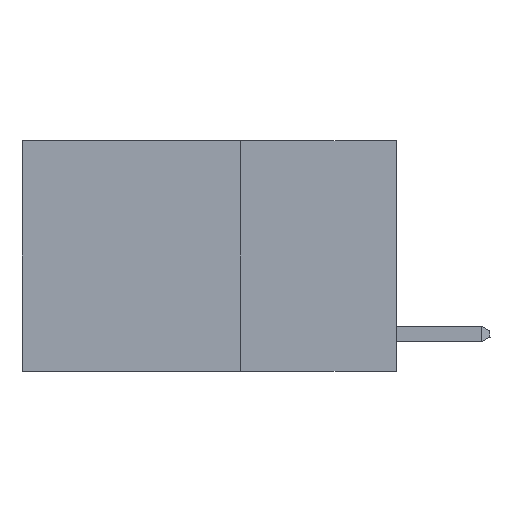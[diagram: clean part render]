
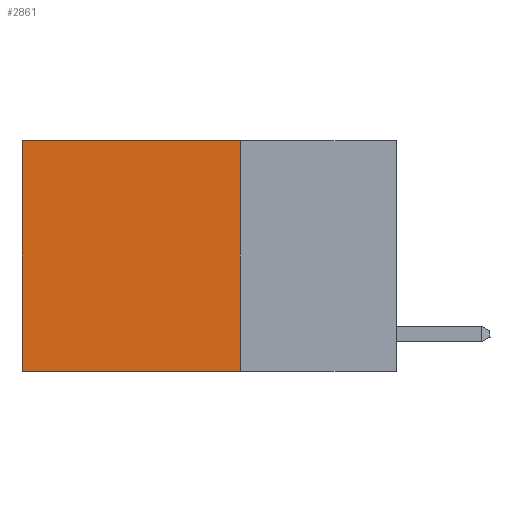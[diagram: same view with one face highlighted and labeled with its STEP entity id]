
A CAD part, left-side view. The second image highlights one B-rep face of the part: STEP entity #2861.
In plain terms, the highlighted planar face has unit normal (-1, 0, 0).
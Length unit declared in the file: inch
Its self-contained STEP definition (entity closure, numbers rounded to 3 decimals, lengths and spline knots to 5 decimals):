
#125 = VERTEX_POINT ( 'NONE', #4732 ) ;
#134 = LINE ( 'NONE', #2473, #5470 ) ;
#230 = ORIENTED_EDGE ( 'NONE', *, *, #5368, .F. ) ;
#691 = VERTEX_POINT ( 'NONE', #4814 ) ;
#1223 = LINE ( 'NONE', #2887, #5284 ) ;
#1435 = CARTESIAN_POINT ( 'NONE',  ( 0.2625, 0.25, -0.37 ) ) ;
#1844 = VERTEX_POINT ( 'NONE', #8013 ) ;
#2473 = CARTESIAN_POINT ( 'NONE',  ( 0.2625, 0.25, 0. ) ) ;
#2756 = LINE ( 'NONE', #1435, #7058 ) ;
#2855 = EDGE_CURVE ( 'NONE', #1844, #125, #134, .T. ) ;
#2861 = ADVANCED_FACE ( 'NONE', ( #9368 ), #5526, .F. ) ;
#2887 = CARTESIAN_POINT ( 'NONE',  ( 0.2625, 0.25, 0. ) ) ;
#3070 = DIRECTION ( 'NONE',  ( 0., 0., -1. ) ) ;
#3236 = CARTESIAN_POINT ( 'NONE',  ( 0.2625, 0.25, 0. ) ) ;
#3537 = EDGE_CURVE ( 'NONE', #691, #5918, #2756, .T. ) ;
#3665 = DIRECTION ( 'NONE',  ( 0., 1., 0. ) ) ;
#3879 = CARTESIAN_POINT ( 'NONE',  ( 0.2625, 0.6, 0. ) ) ;
#3887 = AXIS2_PLACEMENT_3D ( 'NONE', #3236, #6290, #3070 ) ;
#4661 = VECTOR ( 'NONE', #6957, 39.37008 ) ;
#4726 = LINE ( 'NONE', #3879, #4661 ) ;
#4732 = CARTESIAN_POINT ( 'NONE',  ( 0.2625, 0.6, 0. ) ) ;
#4814 = CARTESIAN_POINT ( 'NONE',  ( 0.2625, 0.25, -0.37 ) ) ;
#5284 = VECTOR ( 'NONE', #5802, 39.37008 ) ;
#5368 = EDGE_CURVE ( 'NONE', #1844, #691, #1223, .T. ) ;
#5470 = VECTOR ( 'NONE', #8674, 39.37008 ) ;
#5526 = PLANE ( 'NONE',  #3887 ) ;
#5737 = EDGE_CURVE ( 'NONE', #125, #5918, #4726, .T. ) ;
#5802 = DIRECTION ( 'NONE',  ( 0., 0., -1. ) ) ;
#5832 = EDGE_LOOP ( 'NONE', ( #7825, #8553, #230, #8358 ) ) ;
#5918 = VERTEX_POINT ( 'NONE', #5923 ) ;
#5923 = CARTESIAN_POINT ( 'NONE',  ( 0.2625, 0.6, -0.37 ) ) ;
#6290 = DIRECTION ( 'NONE',  ( 1., 0., 0. ) ) ;
#6957 = DIRECTION ( 'NONE',  ( 0., 0., -1. ) ) ;
#7058 = VECTOR ( 'NONE', #3665, 39.37008 ) ;
#7825 = ORIENTED_EDGE ( 'NONE', *, *, #5737, .T. ) ;
#8013 = CARTESIAN_POINT ( 'NONE',  ( 0.2625, 0.25, 0. ) ) ;
#8358 = ORIENTED_EDGE ( 'NONE', *, *, #2855, .T. ) ;
#8553 = ORIENTED_EDGE ( 'NONE', *, *, #3537, .F. ) ;
#8674 = DIRECTION ( 'NONE',  ( 0., 1., 0. ) ) ;
#9368 = FACE_OUTER_BOUND ( 'NONE', #5832, .T. ) ;
